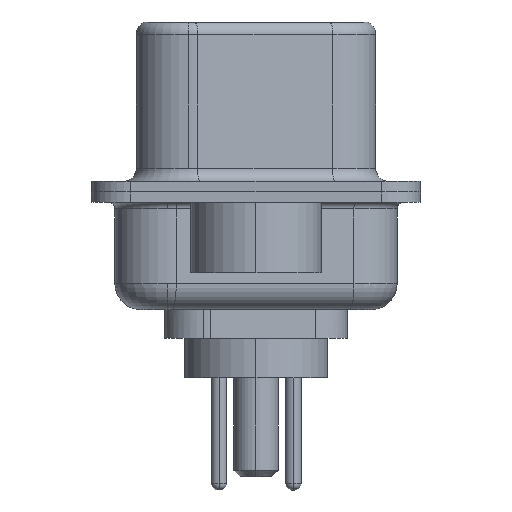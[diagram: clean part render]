
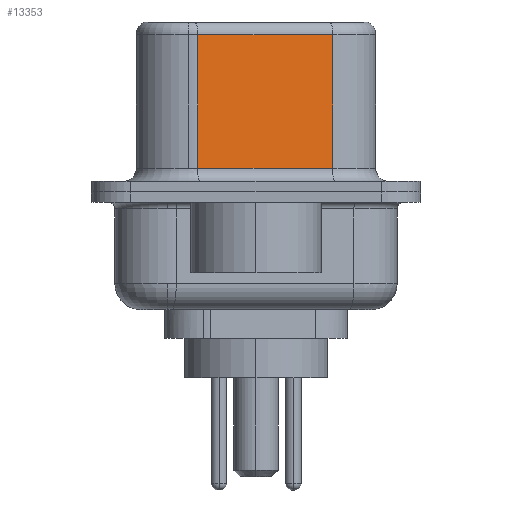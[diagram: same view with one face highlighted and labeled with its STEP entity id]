
A CAD part, left-side view. The second image highlights one B-rep face of the part: STEP entity #13353.
In plain terms, the highlighted planar face has unit normal (-0.985, -0.174, 0).
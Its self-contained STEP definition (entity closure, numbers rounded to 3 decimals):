
#465 = CARTESIAN_POINT ( 'NONE',  ( 4.585, -2.927, 6.02 ) ) ;
#1471 = CARTESIAN_POINT ( 'NONE',  ( 3.675, 2.233, 6.02 ) ) ;
#1545 = LINE ( 'NONE', #15039, #18292 ) ;
#1857 = VECTOR ( 'NONE', #2831, 1000. ) ;
#2831 = DIRECTION ( 'NONE',  ( 0., 0., -1. ) ) ;
#3081 = VECTOR ( 'NONE', #10162, 1000. ) ;
#3206 = CARTESIAN_POINT ( 'NONE',  ( 4.585, -2.927, 6.02 ) ) ;
#3655 = PLANE ( 'NONE',  #5851 ) ;
#4292 = ORIENTED_EDGE ( 'NONE', *, *, #19321, .T. ) ;
#5265 = DIRECTION ( 'NONE',  ( 0.985, 0.174, 0. ) ) ;
#5851 = AXIS2_PLACEMENT_3D ( 'NONE', #14983, #5265, #16690 ) ;
#6091 = LINE ( 'NONE', #12559, #1857 ) ;
#6157 = VERTEX_POINT ( 'NONE', #3206 ) ;
#9257 = ORIENTED_EDGE ( 'NONE', *, *, #20642, .T. ) ;
#9503 = LINE ( 'NONE', #20210, #12318 ) ;
#10095 = EDGE_LOOP ( 'NONE', ( #13611, #4292, #11674, #9257 ) ) ;
#10162 = DIRECTION ( 'NONE',  ( -0.174, 0.985, 0. ) ) ;
#11023 = EDGE_CURVE ( 'NONE', #15195, #19213, #6091, .T. ) ;
#11435 = VERTEX_POINT ( 'NONE', #16978 ) ;
#11674 = ORIENTED_EDGE ( 'NONE', *, *, #11023, .T. ) ;
#12318 = VECTOR ( 'NONE', #20064, 1000. ) ;
#12559 = CARTESIAN_POINT ( 'NONE',  ( 3.675, 2.233, 6.52 ) ) ;
#13353 = ADVANCED_FACE ( 'NONE', ( #17023 ), #3655, .F. ) ;
#13373 = DIRECTION ( 'NONE',  ( 0.174, -0.985, 0. ) ) ;
#13611 = ORIENTED_EDGE ( 'NONE', *, *, #16989, .F. ) ;
#14983 = CARTESIAN_POINT ( 'NONE',  ( 4.585, -2.927, 6.52 ) ) ;
#15039 = CARTESIAN_POINT ( 'NONE',  ( 4.585, -2.927, 0.9 ) ) ;
#15195 = VERTEX_POINT ( 'NONE', #1471 ) ;
#16447 = CARTESIAN_POINT ( 'NONE',  ( 3.675, 2.233, 0.9 ) ) ;
#16690 = DIRECTION ( 'NONE',  ( -0.174, 0.985, 0. ) ) ;
#16978 = CARTESIAN_POINT ( 'NONE',  ( 4.585, -2.927, 0.9 ) ) ;
#16989 = EDGE_CURVE ( 'NONE', #6157, #11435, #9503, .T. ) ;
#17023 = FACE_OUTER_BOUND ( 'NONE', #10095, .T. ) ;
#18292 = VECTOR ( 'NONE', #13373, 1000. ) ;
#19213 = VERTEX_POINT ( 'NONE', #16447 ) ;
#19321 = EDGE_CURVE ( 'NONE', #6157, #15195, #20375, .T. ) ;
#20064 = DIRECTION ( 'NONE',  ( 0., 0., -1. ) ) ;
#20210 = CARTESIAN_POINT ( 'NONE',  ( 4.585, -2.927, 6.52 ) ) ;
#20375 = LINE ( 'NONE', #465, #3081 ) ;
#20642 = EDGE_CURVE ( 'NONE', #19213, #11435, #1545, .T. ) ;
